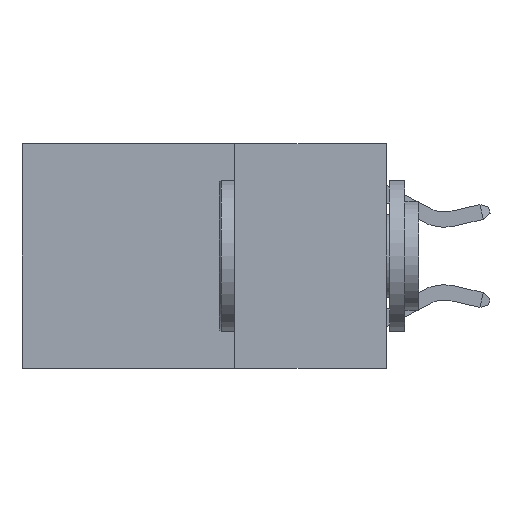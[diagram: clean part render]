
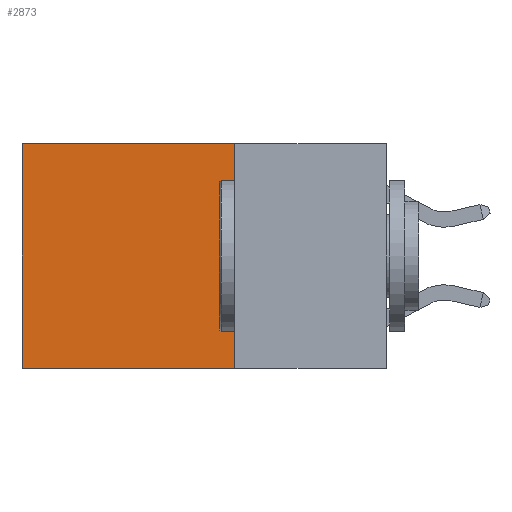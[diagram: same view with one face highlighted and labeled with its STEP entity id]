
A CAD part, left-side view. The second image highlights one B-rep face of the part: STEP entity #2873.
In plain terms, the highlighted planar face has unit normal (-1, 0, 0).
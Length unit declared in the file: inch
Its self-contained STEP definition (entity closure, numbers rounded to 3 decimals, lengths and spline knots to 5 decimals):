
#1 = DIRECTION ( 'NONE',  ( 0., 1., 0. ) ) ;
#1083 = LINE ( 'NONE', #9575, #8781 ) ;
#1632 = LINE ( 'NONE', #8231, #8314 ) ;
#1970 = CARTESIAN_POINT ( 'NONE',  ( 0.2625, 0.6, 0. ) ) ;
#2454 = CARTESIAN_POINT ( 'NONE',  ( 0.2625, 0.25, -0.37 ) ) ;
#2597 = EDGE_CURVE ( 'NONE', #9534, #7057, #5391, .T. ) ;
#2836 = DIRECTION ( 'NONE',  ( 0., 0., -1. ) ) ;
#2873 = ADVANCED_FACE ( 'NONE', ( #11767 ), #12770, .F. ) ;
#3043 = CARTESIAN_POINT ( 'NONE',  ( 0.2625, 0.6, 0. ) ) ;
#3086 = DIRECTION ( 'NONE',  ( 0., 0., -1. ) ) ;
#3424 = ORIENTED_EDGE ( 'NONE', *, *, #2597, .T. ) ;
#3709 = VERTEX_POINT ( 'NONE', #7226 ) ;
#4120 = EDGE_CURVE ( 'NONE', #6636, #7057, #6090, .T. ) ;
#5371 = CARTESIAN_POINT ( 'NONE',  ( 0.2625, 0.25, 0. ) ) ;
#5391 = LINE ( 'NONE', #1970, #7998 ) ;
#6090 = LINE ( 'NONE', #11457, #6792 ) ;
#6346 = EDGE_LOOP ( 'NONE', ( #3424, #12861, #12024, #10521 ) ) ;
#6636 = VERTEX_POINT ( 'NONE', #2454 ) ;
#6792 = VECTOR ( 'NONE', #13683, 39.37008 ) ;
#7057 = VERTEX_POINT ( 'NONE', #10146 ) ;
#7226 = CARTESIAN_POINT ( 'NONE',  ( 0.2625, 0.25, 0. ) ) ;
#7998 = VECTOR ( 'NONE', #3086, 39.37008 ) ;
#8231 = CARTESIAN_POINT ( 'NONE',  ( 0.2625, 0.25, 0. ) ) ;
#8314 = VECTOR ( 'NONE', #13793, 39.37008 ) ;
#8781 = VECTOR ( 'NONE', #1, 39.37008 ) ;
#9397 = AXIS2_PLACEMENT_3D ( 'NONE', #5371, #9787, #2836 ) ;
#9534 = VERTEX_POINT ( 'NONE', #3043 ) ;
#9575 = CARTESIAN_POINT ( 'NONE',  ( 0.2625, 0.25, 0. ) ) ;
#9787 = DIRECTION ( 'NONE',  ( 1., 0., 0. ) ) ;
#10146 = CARTESIAN_POINT ( 'NONE',  ( 0.2625, 0.6, -0.37 ) ) ;
#10521 = ORIENTED_EDGE ( 'NONE', *, *, #13624, .T. ) ;
#11457 = CARTESIAN_POINT ( 'NONE',  ( 0.2625, 0.25, -0.37 ) ) ;
#11767 = FACE_OUTER_BOUND ( 'NONE', #6346, .T. ) ;
#12024 = ORIENTED_EDGE ( 'NONE', *, *, #13293, .F. ) ;
#12770 = PLANE ( 'NONE',  #9397 ) ;
#12861 = ORIENTED_EDGE ( 'NONE', *, *, #4120, .F. ) ;
#13293 = EDGE_CURVE ( 'NONE', #3709, #6636, #1632, .T. ) ;
#13624 = EDGE_CURVE ( 'NONE', #3709, #9534, #1083, .T. ) ;
#13683 = DIRECTION ( 'NONE',  ( 0., 1., 0. ) ) ;
#13793 = DIRECTION ( 'NONE',  ( 0., 0., -1. ) ) ;
